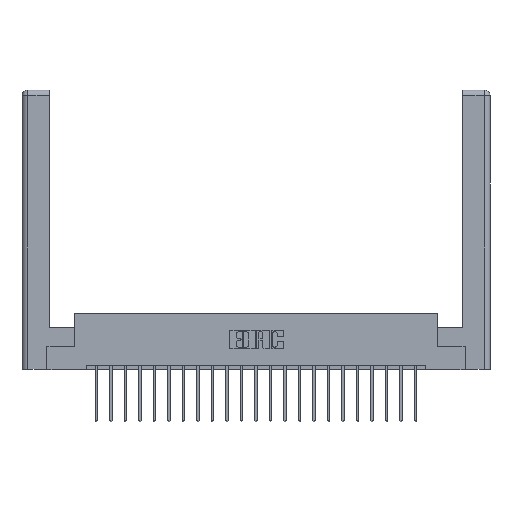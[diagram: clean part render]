
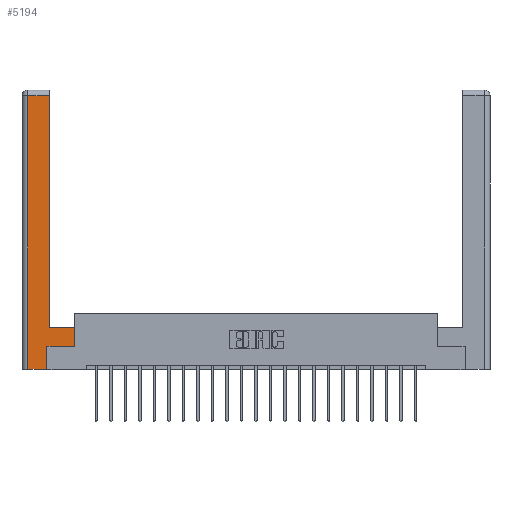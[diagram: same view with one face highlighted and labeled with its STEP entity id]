
A CAD part, top view. The second image highlights one B-rep face of the part: STEP entity #5194.
In plain terms, the highlighted planar face has unit normal (0, 0, 1).
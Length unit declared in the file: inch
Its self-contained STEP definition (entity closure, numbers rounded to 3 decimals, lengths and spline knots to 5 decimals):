
#164 = CARTESIAN_POINT ( 'NONE',  ( 0.265, 0.245, 0. ) ) ;
#760 = DIRECTION ( 'NONE',  ( 1., 0., 0. ) ) ;
#967 = CARTESIAN_POINT ( 'NONE',  ( 0.295, 0.45, 0. ) ) ;
#1060 = LINE ( 'NONE', #3452, #12170 ) ;
#1685 = DIRECTION ( 'NONE',  ( 0., 0., -1. ) ) ;
#2000 = VECTOR ( 'NONE', #11215, 39.37008 ) ;
#2215 = EDGE_CURVE ( 'NONE', #2746, #17564, #6332, .T. ) ;
#2746 = VERTEX_POINT ( 'NONE', #18357 ) ;
#3369 = DIRECTION ( 'NONE',  ( -1., 0., 0. ) ) ;
#3452 = CARTESIAN_POINT ( 'NONE',  ( 0.0615, 2.94, 0. ) ) ;
#3616 = EDGE_CURVE ( 'NONE', #8691, #18709, #17886, .T. ) ;
#3820 = LINE ( 'NONE', #14458, #6341 ) ;
#4424 = DIRECTION ( 'NONE',  ( -1., 0., 0. ) ) ;
#4680 = CARTESIAN_POINT ( 'NONE',  ( 0.565, 0.245, 0. ) ) ;
#4930 = PLANE ( 'NONE',  #19443 ) ;
#5194 = ADVANCED_FACE ( 'NONE', ( #11258 ), #4930, .F. ) ;
#5482 = DIRECTION ( 'NONE',  ( -1., 0., 0. ) ) ;
#5517 = ORIENTED_EDGE ( 'NONE', *, *, #10919, .T. ) ;
#5846 = EDGE_CURVE ( 'NONE', #18709, #9674, #3820, .T. ) ;
#6028 = DIRECTION ( 'NONE',  ( 0., -1., 0. ) ) ;
#6147 = CARTESIAN_POINT ( 'NONE',  ( 0.265, 0., 0. ) ) ;
#6189 = VECTOR ( 'NONE', #6028, 39.37008 ) ;
#6332 = LINE ( 'NONE', #6147, #10525 ) ;
#6341 = VECTOR ( 'NONE', #16177, 39.37008 ) ;
#6451 = CARTESIAN_POINT ( 'NONE',  ( 0.265, 0.245, 0. ) ) ;
#7632 = CARTESIAN_POINT ( 'NONE',  ( 0.295, 3., 0. ) ) ;
#8050 = VECTOR ( 'NONE', #22145, 39.37008 ) ;
#8083 = ORIENTED_EDGE ( 'NONE', *, *, #9701, .T. ) ;
#8691 = VERTEX_POINT ( 'NONE', #164 ) ;
#8988 = VERTEX_POINT ( 'NONE', #967 ) ;
#9085 = CARTESIAN_POINT ( 'NONE',  ( 0.565, 0.45, 0. ) ) ;
#9176 = VECTOR ( 'NONE', #4424, 39.37008 ) ;
#9256 = CARTESIAN_POINT ( 'NONE',  ( 0.565, 0.245, 0. ) ) ;
#9674 = VERTEX_POINT ( 'NONE', #9085 ) ;
#9701 = EDGE_CURVE ( 'NONE', #17914, #2746, #18893, .T. ) ;
#10525 = VECTOR ( 'NONE', #760, 39.37008 ) ;
#10919 = EDGE_CURVE ( 'NONE', #17564, #8691, #11670, .T. ) ;
#11181 = EDGE_CURVE ( 'NONE', #21367, #17914, #1060, .T. ) ;
#11215 = DIRECTION ( 'NONE',  ( 0., 1., 0. ) ) ;
#11258 = FACE_OUTER_BOUND ( 'NONE', #15297, .T. ) ;
#11670 = LINE ( 'NONE', #6451, #8050 ) ;
#11798 = ORIENTED_EDGE ( 'NONE', *, *, #15838, .T. ) ;
#11982 = CARTESIAN_POINT ( 'NONE',  ( 0.0615, 2.94, 0. ) ) ;
#12170 = VECTOR ( 'NONE', #5482, 39.37008 ) ;
#13617 = ORIENTED_EDGE ( 'NONE', *, *, #18173, .T. ) ;
#14406 = CARTESIAN_POINT ( 'NONE',  ( 0.295, 2.94, 0. ) ) ;
#14458 = CARTESIAN_POINT ( 'NONE',  ( 0.565, 0.45, 0. ) ) ;
#14678 = LINE ( 'NONE', #16229, #9176 ) ;
#15297 = EDGE_LOOP ( 'NONE', ( #11798, #20812, #8083, #17921, #5517, #19551, #20107, #13617 ) ) ;
#15614 = CARTESIAN_POINT ( 'NONE',  ( 0., 0., 0. ) ) ;
#15838 = EDGE_CURVE ( 'NONE', #8988, #21367, #16144, .T. ) ;
#16144 = LINE ( 'NONE', #7632, #2000 ) ;
#16177 = DIRECTION ( 'NONE',  ( 0., 1., 0. ) ) ;
#16229 = CARTESIAN_POINT ( 'NONE',  ( 0.295, 0.45, 0. ) ) ;
#16556 = CARTESIAN_POINT ( 'NONE',  ( 0.265, 0., 0. ) ) ;
#16625 = CARTESIAN_POINT ( 'NONE',  ( 0.0615, 0., 0. ) ) ;
#17323 = VECTOR ( 'NONE', #21925, 39.37008 ) ;
#17564 = VERTEX_POINT ( 'NONE', #16556 ) ;
#17886 = LINE ( 'NONE', #4680, #17323 ) ;
#17914 = VERTEX_POINT ( 'NONE', #11982 ) ;
#17921 = ORIENTED_EDGE ( 'NONE', *, *, #2215, .T. ) ;
#18173 = EDGE_CURVE ( 'NONE', #9674, #8988, #14678, .T. ) ;
#18357 = CARTESIAN_POINT ( 'NONE',  ( 0.0615, 0., 0. ) ) ;
#18709 = VERTEX_POINT ( 'NONE', #9256 ) ;
#18893 = LINE ( 'NONE', #16625, #6189 ) ;
#19443 = AXIS2_PLACEMENT_3D ( 'NONE', #15614, #1685, #3369 ) ;
#19551 = ORIENTED_EDGE ( 'NONE', *, *, #3616, .T. ) ;
#20107 = ORIENTED_EDGE ( 'NONE', *, *, #5846, .T. ) ;
#20812 = ORIENTED_EDGE ( 'NONE', *, *, #11181, .T. ) ;
#21367 = VERTEX_POINT ( 'NONE', #14406 ) ;
#21925 = DIRECTION ( 'NONE',  ( 1., 0., 0. ) ) ;
#22145 = DIRECTION ( 'NONE',  ( 0., 1., 0. ) ) ;
